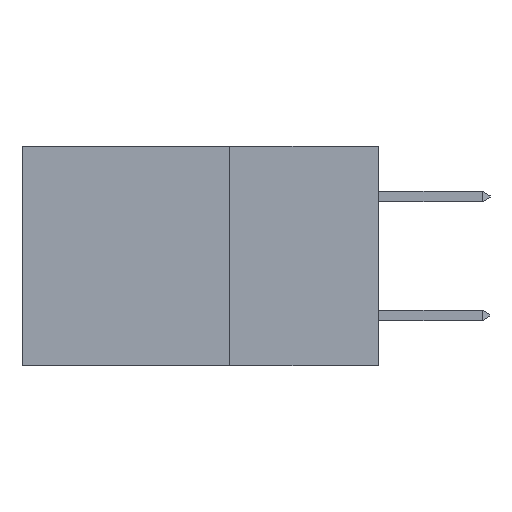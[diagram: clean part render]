
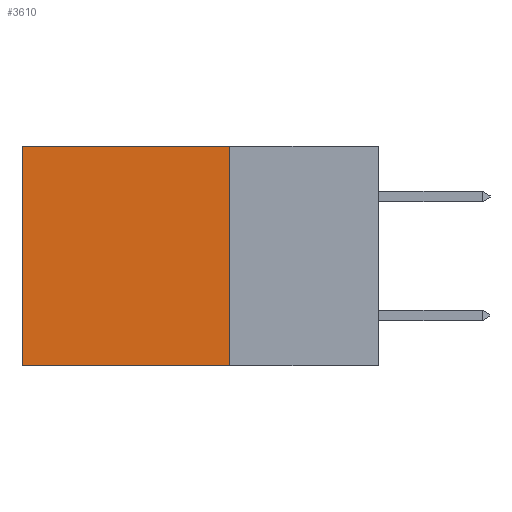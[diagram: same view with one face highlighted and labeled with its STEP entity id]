
A CAD part, left-side view. The second image highlights one B-rep face of the part: STEP entity #3610.
In plain terms, the highlighted planar face has unit normal (-1, 0, 0).
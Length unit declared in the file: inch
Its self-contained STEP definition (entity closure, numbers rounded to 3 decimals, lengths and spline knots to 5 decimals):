
#941 = VECTOR ( 'NONE', #21485, 39.37008 ) ;
#945 = VECTOR ( 'NONE', #16332, 39.37008 ) ;
#1049 = FACE_OUTER_BOUND ( 'NONE', #14235, .T. ) ;
#1521 = LINE ( 'NONE', #6001, #945 ) ;
#2737 = AXIS2_PLACEMENT_3D ( 'NONE', #19590, #18448, #18397 ) ;
#3610 = ADVANCED_FACE ( 'NONE', ( #1049 ), #18746, .F. ) ;
#5717 = LINE ( 'NONE', #21869, #941 ) ;
#6001 = CARTESIAN_POINT ( 'NONE',  ( 0.2615, 0.6, -0.37 ) ) ;
#6091 = CARTESIAN_POINT ( 'NONE',  ( 0.2615, 0.25, 0. ) ) ;
#6351 = VECTOR ( 'NONE', #6640, 39.37008 ) ;
#6528 = EDGE_CURVE ( 'NONE', #13026, #19545, #5717, .T. ) ;
#6640 = DIRECTION ( 'NONE',  ( 0., 1., 0. ) ) ;
#7871 = CARTESIAN_POINT ( 'NONE',  ( 0.2615, 0.6, -0.37 ) ) ;
#8693 = EDGE_CURVE ( 'NONE', #12756, #18061, #10838, .T. ) ;
#9998 = CARTESIAN_POINT ( 'NONE',  ( 0.2615, 0.25, -0.37 ) ) ;
#10838 = LINE ( 'NONE', #13447, #6351 ) ;
#11573 = EDGE_CURVE ( 'NONE', #19545, #18061, #1521, .T. ) ;
#11717 = DIRECTION ( 'NONE',  ( 0., 0., -1. ) ) ;
#11733 = CARTESIAN_POINT ( 'NONE',  ( 0.2615, 0.6, 0. ) ) ;
#12756 = VERTEX_POINT ( 'NONE', #15818 ) ;
#13026 = VERTEX_POINT ( 'NONE', #6091 ) ;
#13237 = EDGE_CURVE ( 'NONE', #13026, #12756, #13404, .T. ) ;
#13404 = LINE ( 'NONE', #9998, #22098 ) ;
#13447 = CARTESIAN_POINT ( 'NONE',  ( 0.2615, 0.25, -0.37 ) ) ;
#13984 = ORIENTED_EDGE ( 'NONE', *, *, #13237, .F. ) ;
#14235 = EDGE_LOOP ( 'NONE', ( #18671, #16588, #13984, #14334 ) ) ;
#14334 = ORIENTED_EDGE ( 'NONE', *, *, #6528, .T. ) ;
#15818 = CARTESIAN_POINT ( 'NONE',  ( 0.2615, 0.25, -0.37 ) ) ;
#16332 = DIRECTION ( 'NONE',  ( 0., 0., -1. ) ) ;
#16588 = ORIENTED_EDGE ( 'NONE', *, *, #8693, .F. ) ;
#18061 = VERTEX_POINT ( 'NONE', #7871 ) ;
#18397 = DIRECTION ( 'NONE',  ( 0., 0., -1. ) ) ;
#18448 = DIRECTION ( 'NONE',  ( 1., 0., 0. ) ) ;
#18671 = ORIENTED_EDGE ( 'NONE', *, *, #11573, .T. ) ;
#18746 = PLANE ( 'NONE',  #2737 ) ;
#19545 = VERTEX_POINT ( 'NONE', #11733 ) ;
#19590 = CARTESIAN_POINT ( 'NONE',  ( 0.2615, 0.25, -0.37 ) ) ;
#21485 = DIRECTION ( 'NONE',  ( 0., 1., 0. ) ) ;
#21869 = CARTESIAN_POINT ( 'NONE',  ( 0.2615, 0.25, 0. ) ) ;
#22098 = VECTOR ( 'NONE', #11717, 39.37008 ) ;
